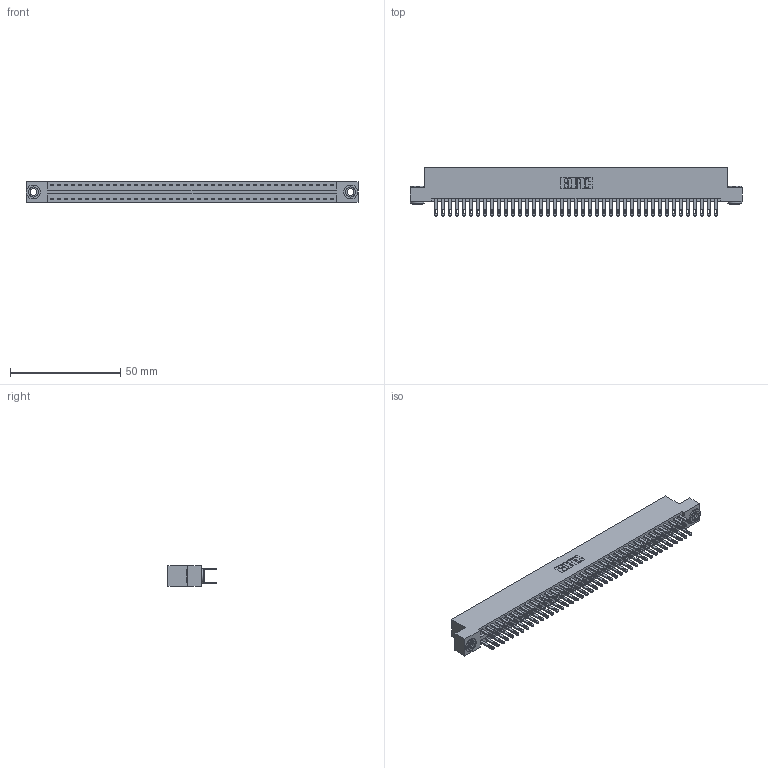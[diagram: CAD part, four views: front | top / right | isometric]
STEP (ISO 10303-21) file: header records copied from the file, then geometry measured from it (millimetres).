
FILE_DESCRIPTION (( 'STEP AP203' ), '1' );
FILE_NAME ('896-082-500-203.STEP', '2021-07-28T02:10:57', ( '' ), ( '' ), 'SwSTEP 2.0', 'SolidWorks 2020', '' );
FILE_SCHEMA (( 'CONFIG_CONTROL_DESIGN' ));
Length unit declared in the file: inch
Products named in the file (4): 345-250-002_345-250-002-102; 896-082-500-203; 345-292-001_345-293-100; 846 Part_Flush Mounting Lugs - 0.156 Dia-TH
Assembly tree (85 placements, depth 2):
  896-082-500-203
    846 Part_Flush Mounting Lugs - 0.156 Dia-TH
    345-292-001_345-293-100  x82
    345-250-002_345-250-002-102  x2
Bounding box: 150.75 x 21.84 x 9.4 mm (x, y, z)
Volume: 14962.1 mm3; surface area: 21623.1 mm2
Topology: 85 solids, 85 shells, 4096 faces, 12459 edges, 8302 vertices
Faces by surface type: plane 2464, cylinder 1624, cone 8
Entity records: 27472 total; most frequent: CARTESIAN_POINT 4503, ORIENTED_EDGE 4430, DIRECTION 4053, EDGE_CURVE 2215, VECTOR 1891, LINE 1891, VERTEX_POINT 1474, AXIS2_PLACEMENT_3D 1081
